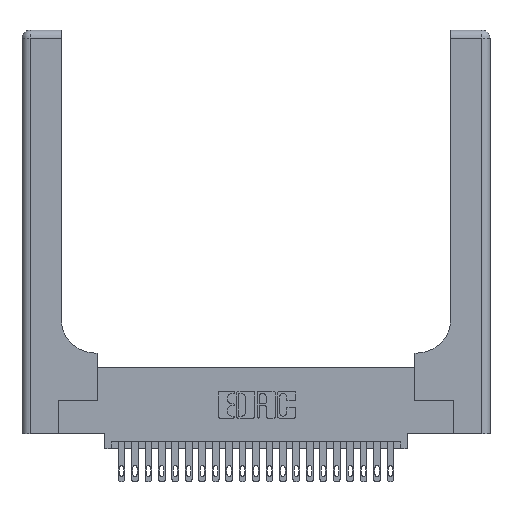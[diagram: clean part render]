
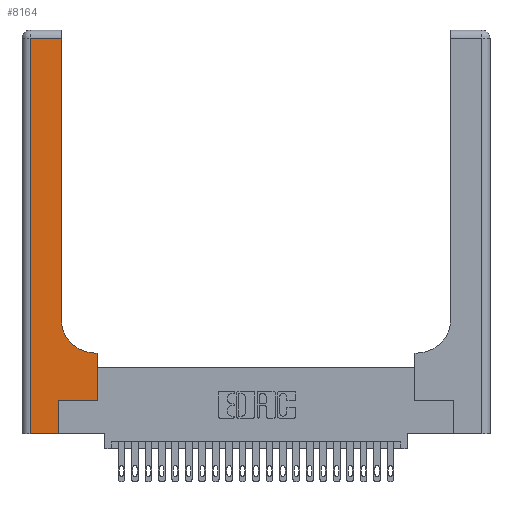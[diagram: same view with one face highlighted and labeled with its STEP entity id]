
A CAD part, top view. The second image highlights one B-rep face of the part: STEP entity #8164.
In plain terms, the highlighted planar face has unit normal (0, 0, 1).
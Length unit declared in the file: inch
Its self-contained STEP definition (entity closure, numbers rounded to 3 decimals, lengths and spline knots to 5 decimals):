
#396 = VECTOR ( 'NONE', #837, 39.37008 ) ;
#741 = LINE ( 'NONE', #3406, #15350 ) ;
#837 = DIRECTION ( 'NONE',  ( -1., 0., 0. ) ) ;
#1297 = ORIENTED_EDGE ( 'NONE', *, *, #15233, .T. ) ;
#1309 = VECTOR ( 'NONE', #12980, 39.37008 ) ;
#1497 = VERTEX_POINT ( 'NONE', #16704 ) ;
#2862 = VERTEX_POINT ( 'NONE', #19034 ) ;
#3406 = CARTESIAN_POINT ( 'NONE',  ( 0.5585, 0.25, 0.37 ) ) ;
#3657 = CARTESIAN_POINT ( 'NONE',  ( 0.269, 0., 0.37 ) ) ;
#3772 = AXIS2_PLACEMENT_3D ( 'NONE', #4602, #14848, #9011 ) ;
#4602 = CARTESIAN_POINT ( 'NONE',  ( 0.5415, 0.85, 0.37 ) ) ;
#4778 = CARTESIAN_POINT ( 'NONE',  ( 0.2915, 2.94, 0.37 ) ) ;
#5153 = ORIENTED_EDGE ( 'NONE', *, *, #12352, .T. ) ;
#5491 = ORIENTED_EDGE ( 'NONE', *, *, #20021, .T. ) ;
#5952 = VECTOR ( 'NONE', #18159, 39.37008 ) ;
#6181 = EDGE_CURVE ( 'NONE', #15666, #2862, #741, .T. ) ;
#6668 = CARTESIAN_POINT ( 'NONE',  ( 0.2915, 0.6, 0.37 ) ) ;
#7259 = VECTOR ( 'NONE', #11561, 39.37008 ) ;
#7376 = PLANE ( 'NONE',  #11363 ) ;
#7458 = DIRECTION ( 'NONE',  ( 0., 1., 0. ) ) ;
#7577 = CARTESIAN_POINT ( 'NONE',  ( 0.5585, 0.25, 0.37 ) ) ;
#7676 = VERTEX_POINT ( 'NONE', #4778 ) ;
#8164 = ADVANCED_FACE ( 'NONE', ( #24405 ), #7376, .F. ) ;
#8525 = LINE ( 'NONE', #23653, #16568 ) ;
#9011 = DIRECTION ( 'NONE',  ( 1., 0., 0. ) ) ;
#9153 = CARTESIAN_POINT ( 'NONE',  ( 0., 2.94, 0.37 ) ) ;
#9679 = EDGE_CURVE ( 'NONE', #9756, #7676, #22735, .T. ) ;
#9756 = VERTEX_POINT ( 'NONE', #11417 ) ;
#10441 = CARTESIAN_POINT ( 'NONE',  ( 0.06, 3., 0.37 ) ) ;
#10852 = EDGE_LOOP ( 'NONE', ( #14310, #22788, #17105, #5491, #15778, #5153, #19542, #1297, #14789 ) ) ;
#11093 = CARTESIAN_POINT ( 'NONE',  ( 0.06, 0., 0.37 ) ) ;
#11107 = CARTESIAN_POINT ( 'NONE',  ( 0.2915, 3., 0.37 ) ) ;
#11131 = LINE ( 'NONE', #6668, #396 ) ;
#11181 = DIRECTION ( 'NONE',  ( 0., 0., -1. ) ) ;
#11363 = AXIS2_PLACEMENT_3D ( 'NONE', #22355, #11181, #14881 ) ;
#11413 = LINE ( 'NONE', #9153, #1309 ) ;
#11417 = CARTESIAN_POINT ( 'NONE',  ( 0.2915, 0.85, 0.37 ) ) ;
#11561 = DIRECTION ( 'NONE',  ( 1., 0., 0. ) ) ;
#12000 = CIRCLE ( 'NONE', #3772, 0.25 ) ;
#12071 = EDGE_CURVE ( 'NONE', #15808, #9756, #12000, .T. ) ;
#12352 = EDGE_CURVE ( 'NONE', #17504, #15666, #17052, .T. ) ;
#12980 = DIRECTION ( 'NONE',  ( -1., 0., 0. ) ) ;
#13628 = CARTESIAN_POINT ( 'NONE',  ( 0.269, 0.25, 0.37 ) ) ;
#14071 = DIRECTION ( 'NONE',  ( 1., 0., 0. ) ) ;
#14232 = EDGE_CURVE ( 'NONE', #1497, #17059, #15776, .T. ) ;
#14310 = ORIENTED_EDGE ( 'NONE', *, *, #9679, .T. ) ;
#14789 = ORIENTED_EDGE ( 'NONE', *, *, #12071, .T. ) ;
#14843 = VERTEX_POINT ( 'NONE', #20418 ) ;
#14848 = DIRECTION ( 'NONE',  ( 0., 0., -1. ) ) ;
#14881 = DIRECTION ( 'NONE',  ( -1., 0., 0. ) ) ;
#15233 = EDGE_CURVE ( 'NONE', #2862, #15808, #11131, .T. ) ;
#15350 = VECTOR ( 'NONE', #20248, 39.37008 ) ;
#15666 = VERTEX_POINT ( 'NONE', #7577 ) ;
#15776 = LINE ( 'NONE', #10441, #5952 ) ;
#15778 = ORIENTED_EDGE ( 'NONE', *, *, #16493, .T. ) ;
#15808 = VERTEX_POINT ( 'NONE', #18957 ) ;
#16493 = EDGE_CURVE ( 'NONE', #14843, #17504, #21069, .T. ) ;
#16568 = VECTOR ( 'NONE', #14071, 39.37008 ) ;
#16704 = CARTESIAN_POINT ( 'NONE',  ( 0.06, 2.94, 0.37 ) ) ;
#16934 = DIRECTION ( 'NONE',  ( 0., 1., 0. ) ) ;
#17052 = LINE ( 'NONE', #13628, #7259 ) ;
#17059 = VERTEX_POINT ( 'NONE', #11093 ) ;
#17105 = ORIENTED_EDGE ( 'NONE', *, *, #14232, .T. ) ;
#17504 = VERTEX_POINT ( 'NONE', #20152 ) ;
#17848 = VECTOR ( 'NONE', #16934, 39.37008 ) ;
#18159 = DIRECTION ( 'NONE',  ( 0., -1., 0. ) ) ;
#18957 = CARTESIAN_POINT ( 'NONE',  ( 0.5415, 0.6, 0.37 ) ) ;
#19034 = CARTESIAN_POINT ( 'NONE',  ( 0.5585, 0.6, 0.37 ) ) ;
#19542 = ORIENTED_EDGE ( 'NONE', *, *, #6181, .T. ) ;
#20021 = EDGE_CURVE ( 'NONE', #17059, #14843, #8525, .T. ) ;
#20152 = CARTESIAN_POINT ( 'NONE',  ( 0.269, 0.25, 0.37 ) ) ;
#20248 = DIRECTION ( 'NONE',  ( 0., 1., 0. ) ) ;
#20418 = CARTESIAN_POINT ( 'NONE',  ( 0.269, 0., 0.37 ) ) ;
#21069 = LINE ( 'NONE', #3657, #17848 ) ;
#21333 = EDGE_CURVE ( 'NONE', #7676, #1497, #11413, .T. ) ;
#21859 = VECTOR ( 'NONE', #7458, 39.37008 ) ;
#22355 = CARTESIAN_POINT ( 'NONE',  ( 0., 3., 0.37 ) ) ;
#22735 = LINE ( 'NONE', #11107, #21859 ) ;
#22788 = ORIENTED_EDGE ( 'NONE', *, *, #21333, .T. ) ;
#23653 = CARTESIAN_POINT ( 'NONE',  ( 0., 0., 0.37 ) ) ;
#24405 = FACE_OUTER_BOUND ( 'NONE', #10852, .T. ) ;
